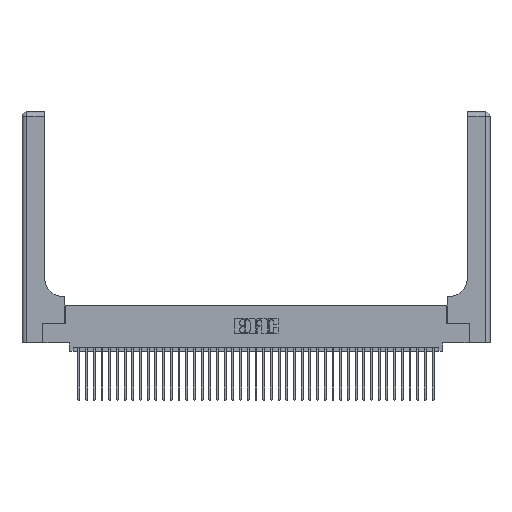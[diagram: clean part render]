
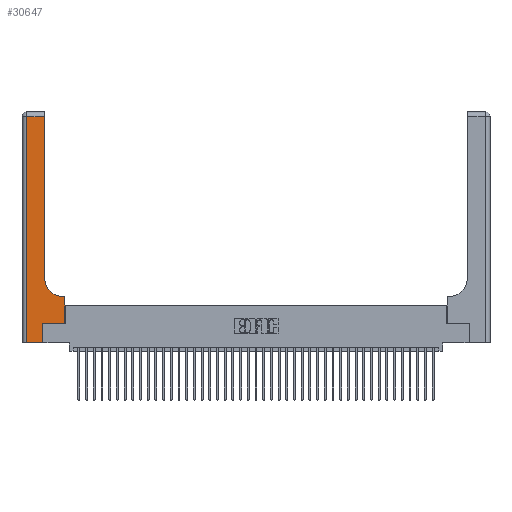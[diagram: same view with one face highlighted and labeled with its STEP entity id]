
A CAD part, top view. The second image highlights one B-rep face of the part: STEP entity #30647.
In plain terms, the highlighted planar face has unit normal (0, 0, 1).
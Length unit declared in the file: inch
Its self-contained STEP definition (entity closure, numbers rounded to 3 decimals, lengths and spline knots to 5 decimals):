
#309 = CIRCLE ( 'NONE', #34554, 0.25 ) ;
#312 = LINE ( 'NONE', #28063, #7985 ) ;
#1531 = EDGE_CURVE ( 'NONE', #35440, #32720, #11119, .T. ) ;
#1626 = VERTEX_POINT ( 'NONE', #20539 ) ;
#2280 = ORIENTED_EDGE ( 'NONE', *, *, #14682, .T. ) ;
#2393 = VERTEX_POINT ( 'NONE', #22892 ) ;
#3062 = EDGE_CURVE ( 'NONE', #22423, #35440, #32489, .T. ) ;
#3356 = LINE ( 'NONE', #4548, #36471 ) ;
#3771 = EDGE_CURVE ( 'NONE', #2393, #14630, #309, .T. ) ;
#4173 = VERTEX_POINT ( 'NONE', #11709 ) ;
#4548 = CARTESIAN_POINT ( 'NONE',  ( 0.5585, 0.25, 0.37 ) ) ;
#4748 = CARTESIAN_POINT ( 'NONE',  ( 0.2915, 0.6, 0.37 ) ) ;
#7209 = EDGE_CURVE ( 'NONE', #1626, #4173, #3356, .T. ) ;
#7965 = VERTEX_POINT ( 'NONE', #20979 ) ;
#7985 = VECTOR ( 'NONE', #9017, 39.37008 ) ;
#9017 = DIRECTION ( 'NONE',  ( 0., 1., 0. ) ) ;
#10650 = CARTESIAN_POINT ( 'NONE',  ( 0.2915, 2.94, 0.37 ) ) ;
#11053 = DIRECTION ( 'NONE',  ( 0., 1., 0. ) ) ;
#11119 = LINE ( 'NONE', #26128, #35611 ) ;
#11248 = DIRECTION ( 'NONE',  ( -1., 0., 0. ) ) ;
#11709 = CARTESIAN_POINT ( 'NONE',  ( 0.5585, 0.6, 0.37 ) ) ;
#11957 = DIRECTION ( 'NONE',  ( -1., 0., 0. ) ) ;
#11963 = LINE ( 'NONE', #4748, #27981 ) ;
#12172 = VECTOR ( 'NONE', #37416, 39.37008 ) ;
#13123 = CARTESIAN_POINT ( 'NONE',  ( 0.5415, 0.85, 0.37 ) ) ;
#14546 = EDGE_CURVE ( 'NONE', #28352, #1626, #30189, .T. ) ;
#14630 = VERTEX_POINT ( 'NONE', #15640 ) ;
#14682 = EDGE_CURVE ( 'NONE', #7965, #28352, #31656, .T. ) ;
#14694 = VECTOR ( 'NONE', #18995, 39.37008 ) ;
#15536 = VECTOR ( 'NONE', #25922, 39.37008 ) ;
#15547 = EDGE_LOOP ( 'NONE', ( #32330, #24667, #21841, #15636, #2280, #26627, #26823, #29397, #35320 ) ) ;
#15636 = ORIENTED_EDGE ( 'NONE', *, *, #25608, .T. ) ;
#15640 = CARTESIAN_POINT ( 'NONE',  ( 0.2915, 0.85, 0.37 ) ) ;
#16288 = AXIS2_PLACEMENT_3D ( 'NONE', #24712, #31107, #11957 ) ;
#16362 = DIRECTION ( 'NONE',  ( 1., 0., 0. ) ) ;
#16538 = EDGE_CURVE ( 'NONE', #14630, #22423, #312, .T. ) ;
#16942 = DIRECTION ( 'NONE',  ( 1., 0., 0. ) ) ;
#18317 = CARTESIAN_POINT ( 'NONE',  ( 0.269, 0.25, 0.37 ) ) ;
#18995 = DIRECTION ( 'NONE',  ( 0., 1., 0. ) ) ;
#19347 = FACE_OUTER_BOUND ( 'NONE', #15547, .T. ) ;
#19735 = VECTOR ( 'NONE', #16942, 39.37008 ) ;
#20539 = CARTESIAN_POINT ( 'NONE',  ( 0.5585, 0.25, 0.37 ) ) ;
#20979 = CARTESIAN_POINT ( 'NONE',  ( 0.269, 0., 0.37 ) ) ;
#21841 = ORIENTED_EDGE ( 'NONE', *, *, #1531, .T. ) ;
#22423 = VERTEX_POINT ( 'NONE', #10650 ) ;
#22703 = CARTESIAN_POINT ( 'NONE',  ( 0., 2.94, 0.37 ) ) ;
#22892 = CARTESIAN_POINT ( 'NONE',  ( 0.5415, 0.6, 0.37 ) ) ;
#24667 = ORIENTED_EDGE ( 'NONE', *, *, #3062, .T. ) ;
#24712 = CARTESIAN_POINT ( 'NONE',  ( 0., 3., 0.37 ) ) ;
#25608 = EDGE_CURVE ( 'NONE', #32720, #7965, #36703, .T. ) ;
#25922 = DIRECTION ( 'NONE',  ( -1., 0., 0. ) ) ;
#26128 = CARTESIAN_POINT ( 'NONE',  ( 0.06, 3., 0.37 ) ) ;
#26627 = ORIENTED_EDGE ( 'NONE', *, *, #14546, .T. ) ;
#26823 = ORIENTED_EDGE ( 'NONE', *, *, #7209, .T. ) ;
#27901 = PLANE ( 'NONE',  #16288 ) ;
#27981 = VECTOR ( 'NONE', #11248, 39.37008 ) ;
#28063 = CARTESIAN_POINT ( 'NONE',  ( 0.2915, 3., 0.37 ) ) ;
#28352 = VERTEX_POINT ( 'NONE', #38624 ) ;
#29397 = ORIENTED_EDGE ( 'NONE', *, *, #38029, .T. ) ;
#30189 = LINE ( 'NONE', #18317, #12172 ) ;
#30591 = CARTESIAN_POINT ( 'NONE',  ( 0.06, 2.94, 0.37 ) ) ;
#30647 = ADVANCED_FACE ( 'NONE', ( #19347 ), #27901, .F. ) ;
#31107 = DIRECTION ( 'NONE',  ( 0., 0., -1. ) ) ;
#31656 = LINE ( 'NONE', #31671, #14694 ) ;
#31671 = CARTESIAN_POINT ( 'NONE',  ( 0.269, 0., 0.37 ) ) ;
#32330 = ORIENTED_EDGE ( 'NONE', *, *, #16538, .T. ) ;
#32489 = LINE ( 'NONE', #22703, #15536 ) ;
#32720 = VERTEX_POINT ( 'NONE', #34145 ) ;
#34145 = CARTESIAN_POINT ( 'NONE',  ( 0.06, 0., 0.37 ) ) ;
#34554 = AXIS2_PLACEMENT_3D ( 'NONE', #13123, #35480, #16362 ) ;
#35320 = ORIENTED_EDGE ( 'NONE', *, *, #3771, .T. ) ;
#35440 = VERTEX_POINT ( 'NONE', #30591 ) ;
#35480 = DIRECTION ( 'NONE',  ( 0., 0., -1. ) ) ;
#35611 = VECTOR ( 'NONE', #38918, 39.37008 ) ;
#36471 = VECTOR ( 'NONE', #11053, 39.37008 ) ;
#36703 = LINE ( 'NONE', #39239, #19735 ) ;
#37416 = DIRECTION ( 'NONE',  ( 1., 0., 0. ) ) ;
#38029 = EDGE_CURVE ( 'NONE', #4173, #2393, #11963, .T. ) ;
#38624 = CARTESIAN_POINT ( 'NONE',  ( 0.269, 0.25, 0.37 ) ) ;
#38918 = DIRECTION ( 'NONE',  ( 0., -1., 0. ) ) ;
#39239 = CARTESIAN_POINT ( 'NONE',  ( 0., 0., 0.37 ) ) ;
